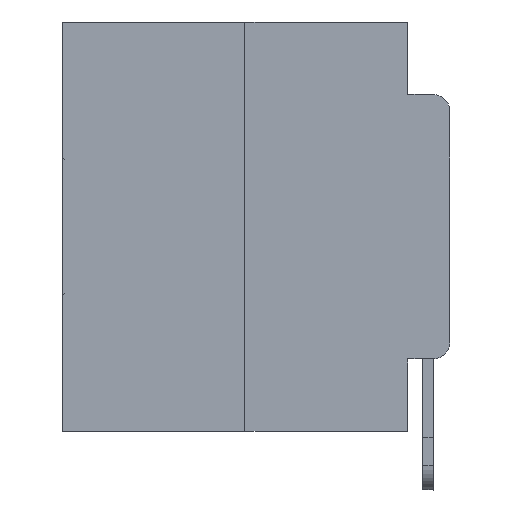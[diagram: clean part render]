
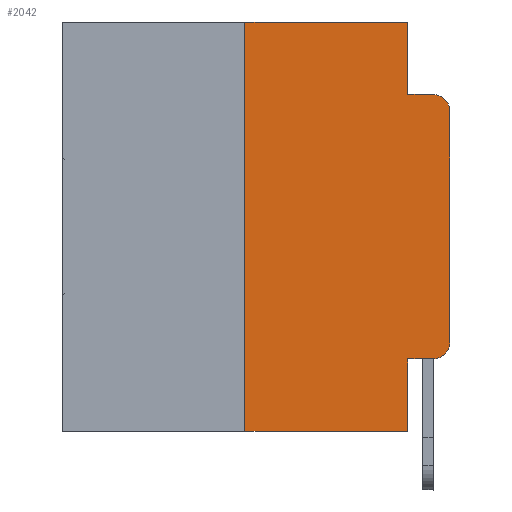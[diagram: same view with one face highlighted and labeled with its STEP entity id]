
A CAD part, left-side view. The second image highlights one B-rep face of the part: STEP entity #2042.
In plain terms, the highlighted planar face has unit normal (-1, 0, 0).
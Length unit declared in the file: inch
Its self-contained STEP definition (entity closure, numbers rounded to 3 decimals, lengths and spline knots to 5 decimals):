
#347 = DIRECTION ( 'NONE',  ( 0., 0., 1. ) ) ;
#463 = PLANE ( 'NONE',  #3968 ) ;
#1841 = DIRECTION ( 'NONE',  ( 0., 0., -1. ) ) ;
#1869 = EDGE_CURVE ( 'NONE', #10127, #28520, #4030, .T. ) ;
#2042 = ADVANCED_FACE ( 'NONE', ( #22845 ), #463, .F. ) ;
#2085 = CARTESIAN_POINT ( 'NONE',  ( 0., 0., 0. ) ) ;
#2442 = DIRECTION ( 'NONE',  ( 0., 0., -1. ) ) ;
#3222 = ORIENTED_EDGE ( 'NONE', *, *, #11781, .T. ) ;
#3424 = ORIENTED_EDGE ( 'NONE', *, *, #21317, .F. ) ;
#3968 = AXIS2_PLACEMENT_3D ( 'NONE', #20624, #13827, #27594 ) ;
#4030 = LINE ( 'NONE', #22415, #16311 ) ;
#4044 = VERTEX_POINT ( 'NONE', #17894 ) ;
#4242 = VERTEX_POINT ( 'NONE', #11803 ) ;
#4469 = DIRECTION ( 'NONE',  ( 0., 0., 1. ) ) ;
#4814 = LINE ( 'NONE', #13726, #18992 ) ;
#4921 = EDGE_LOOP ( 'NONE', ( #21861, #5183, #3424, #22502, #18531, #10506, #3222, #26868, #11245, #22846 ) ) ;
#5183 = ORIENTED_EDGE ( 'NONE', *, *, #8612, .T. ) ;
#6845 = LINE ( 'NONE', #25502, #12726 ) ;
#7171 = CARTESIAN_POINT ( 'NONE',  ( 0., 0.051, -0.4115 ) ) ;
#7578 = AXIS2_PLACEMENT_3D ( 'NONE', #11932, #9719, #25562 ) ;
#8585 = CIRCLE ( 'NONE', #12358, 0.02 ) ;
#8612 = EDGE_CURVE ( 'NONE', #27683, #10200, #8585, .T. ) ;
#8764 = EDGE_CURVE ( 'NONE', #4044, #4242, #4814, .T. ) ;
#9719 = DIRECTION ( 'NONE',  ( -1., 0., 0. ) ) ;
#9915 = VECTOR ( 'NONE', #18143, 39.37008 ) ;
#10127 = VERTEX_POINT ( 'NONE', #18876 ) ;
#10200 = VERTEX_POINT ( 'NONE', #28498 ) ;
#10274 = VECTOR ( 'NONE', #25915, 39.37008 ) ;
#10397 = CARTESIAN_POINT ( 'NONE',  ( 0., 0., -0.3915 ) ) ;
#10506 = ORIENTED_EDGE ( 'NONE', *, *, #8764, .F. ) ;
#10682 = LINE ( 'NONE', #28923, #24267 ) ;
#10909 = CARTESIAN_POINT ( 'NONE',  ( 0., 0.02, -0.1085 ) ) ;
#11245 = ORIENTED_EDGE ( 'NONE', *, *, #14435, .T. ) ;
#11386 = CIRCLE ( 'NONE', #7578, 0.02 ) ;
#11781 = EDGE_CURVE ( 'NONE', #4044, #21340, #10682, .T. ) ;
#11803 = CARTESIAN_POINT ( 'NONE',  ( 0., 0.25, 0. ) ) ;
#11895 = CARTESIAN_POINT ( 'NONE',  ( 0., 0.051, -0.4115 ) ) ;
#11932 = CARTESIAN_POINT ( 'NONE',  ( 0., 0.02, -0.3915 ) ) ;
#12292 = LINE ( 'NONE', #26352, #10274 ) ;
#12358 = AXIS2_PLACEMENT_3D ( 'NONE', #10909, #29132, #1841 ) ;
#12726 = VECTOR ( 'NONE', #23271, 39.37008 ) ;
#12761 = EDGE_CURVE ( 'NONE', #20706, #21340, #13738, .T. ) ;
#13726 = CARTESIAN_POINT ( 'NONE',  ( 0., 0.25, 0. ) ) ;
#13738 = LINE ( 'NONE', #22762, #19757 ) ;
#13827 = DIRECTION ( 'NONE',  ( 1., 0., 0. ) ) ;
#14435 = EDGE_CURVE ( 'NONE', #20706, #19865, #20361, .T. ) ;
#16311 = VECTOR ( 'NONE', #24776, 39.37008 ) ;
#17129 = EDGE_CURVE ( 'NONE', #19865, #20772, #11386, .T. ) ;
#17894 = CARTESIAN_POINT ( 'NONE',  ( 0., 0.25, -0.5 ) ) ;
#18026 = CARTESIAN_POINT ( 'NONE',  ( 0., 0.051, -0.0885 ) ) ;
#18143 = DIRECTION ( 'NONE',  ( 0., -1., 0. ) ) ;
#18531 = ORIENTED_EDGE ( 'NONE', *, *, #25267, .F. ) ;
#18876 = CARTESIAN_POINT ( 'NONE',  ( 0., 0.051, 0. ) ) ;
#18992 = VECTOR ( 'NONE', #347, 39.37008 ) ;
#19301 = VECTOR ( 'NONE', #4469, 39.37008 ) ;
#19637 = CARTESIAN_POINT ( 'NONE',  ( 0., 0.02, -0.4115 ) ) ;
#19757 = VECTOR ( 'NONE', #2442, 39.37008 ) ;
#19865 = VERTEX_POINT ( 'NONE', #19637 ) ;
#20361 = LINE ( 'NONE', #7171, #9915 ) ;
#20624 = CARTESIAN_POINT ( 'NONE',  ( 0., 0.473, 0. ) ) ;
#20706 = VERTEX_POINT ( 'NONE', #11895 ) ;
#20772 = VERTEX_POINT ( 'NONE', #10397 ) ;
#21062 = CARTESIAN_POINT ( 'NONE',  ( 0., 0., -0.1085 ) ) ;
#21317 = EDGE_CURVE ( 'NONE', #28520, #10200, #12292, .T. ) ;
#21340 = VERTEX_POINT ( 'NONE', #23431 ) ;
#21861 = ORIENTED_EDGE ( 'NONE', *, *, #22285, .T. ) ;
#22285 = EDGE_CURVE ( 'NONE', #20772, #27683, #22691, .T. ) ;
#22415 = CARTESIAN_POINT ( 'NONE',  ( 0., 0.051, 0. ) ) ;
#22502 = ORIENTED_EDGE ( 'NONE', *, *, #1869, .F. ) ;
#22691 = LINE ( 'NONE', #2085, #19301 ) ;
#22762 = CARTESIAN_POINT ( 'NONE',  ( 0., 0.051, 0. ) ) ;
#22845 = FACE_OUTER_BOUND ( 'NONE', #4921, .T. ) ;
#22846 = ORIENTED_EDGE ( 'NONE', *, *, #17129, .T. ) ;
#23271 = DIRECTION ( 'NONE',  ( 0., -1., 0. ) ) ;
#23431 = CARTESIAN_POINT ( 'NONE',  ( 0., 0.051, -0.5 ) ) ;
#24267 = VECTOR ( 'NONE', #29070, 39.37008 ) ;
#24776 = DIRECTION ( 'NONE',  ( 0., 0., -1. ) ) ;
#25267 = EDGE_CURVE ( 'NONE', #4242, #10127, #6845, .T. ) ;
#25502 = CARTESIAN_POINT ( 'NONE',  ( 0., 0.473, 0. ) ) ;
#25562 = DIRECTION ( 'NONE',  ( 0., 0., -1. ) ) ;
#25915 = DIRECTION ( 'NONE',  ( 0., -1., 0. ) ) ;
#26352 = CARTESIAN_POINT ( 'NONE',  ( 0., 0.051, -0.0885 ) ) ;
#26868 = ORIENTED_EDGE ( 'NONE', *, *, #12761, .F. ) ;
#27594 = DIRECTION ( 'NONE',  ( 0., 0., -1. ) ) ;
#27683 = VERTEX_POINT ( 'NONE', #21062 ) ;
#28498 = CARTESIAN_POINT ( 'NONE',  ( 0., 0.02, -0.0885 ) ) ;
#28520 = VERTEX_POINT ( 'NONE', #18026 ) ;
#28923 = CARTESIAN_POINT ( 'NONE',  ( 0., 0.473, -0.5 ) ) ;
#29070 = DIRECTION ( 'NONE',  ( 0., -1., 0. ) ) ;
#29132 = DIRECTION ( 'NONE',  ( -1., 0., 0. ) ) ;
